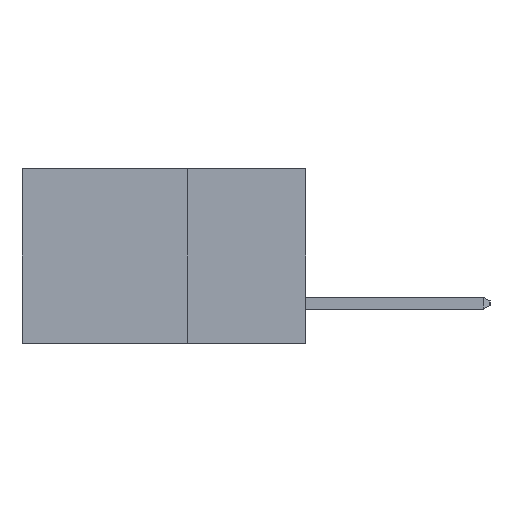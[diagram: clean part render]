
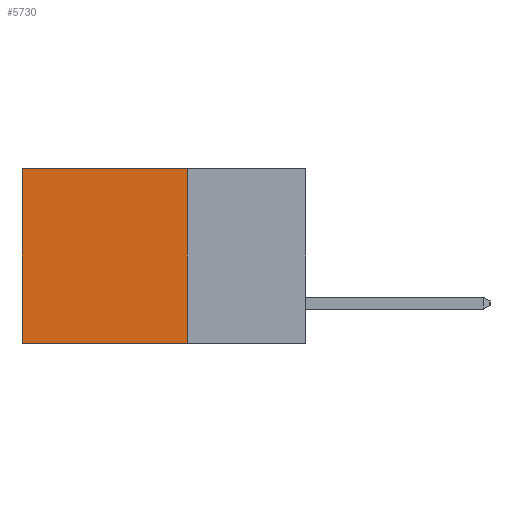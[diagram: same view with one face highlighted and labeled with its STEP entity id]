
A CAD part, left-side view. The second image highlights one B-rep face of the part: STEP entity #5730.
In plain terms, the highlighted planar face has unit normal (-1, 0, 0).
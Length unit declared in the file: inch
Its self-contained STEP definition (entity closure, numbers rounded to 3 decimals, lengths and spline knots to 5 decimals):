
#432 = ORIENTED_EDGE ( 'NONE', *, *, #12054, .F. ) ;
#1038 = EDGE_LOOP ( 'NONE', ( #14572, #3369, #432, #4384 ) ) ;
#1232 = CARTESIAN_POINT ( 'NONE',  ( 0.298, 0.25, 0. ) ) ;
#1444 = VECTOR ( 'NONE', #12503, 39.37008 ) ;
#2097 = CARTESIAN_POINT ( 'NONE',  ( 0.298, 0.6, -0.37 ) ) ;
#2151 = VERTEX_POINT ( 'NONE', #5497 ) ;
#2325 = LINE ( 'NONE', #1232, #12451 ) ;
#2976 = DIRECTION ( 'NONE',  ( 0., 0., -1. ) ) ;
#3150 = EDGE_CURVE ( 'NONE', #10001, #14254, #14470, .T. ) ;
#3329 = CARTESIAN_POINT ( 'NONE',  ( 0.298, 0.25, -0.37 ) ) ;
#3369 = ORIENTED_EDGE ( 'NONE', *, *, #3150, .F. ) ;
#4040 = CARTESIAN_POINT ( 'NONE',  ( 0.298, 0.25, 0. ) ) ;
#4271 = CARTESIAN_POINT ( 'NONE',  ( 0.298, 0.6, 0. ) ) ;
#4372 = DIRECTION ( 'NONE',  ( 1., 0., 0. ) ) ;
#4384 = ORIENTED_EDGE ( 'NONE', *, *, #6119, .T. ) ;
#5010 = LINE ( 'NONE', #4040, #14795 ) ;
#5497 = CARTESIAN_POINT ( 'NONE',  ( 0.298, 0.6, 0. ) ) ;
#5730 = ADVANCED_FACE ( 'NONE', ( #5785 ), #10461, .F. ) ;
#5785 = FACE_OUTER_BOUND ( 'NONE', #1038, .T. ) ;
#6119 = EDGE_CURVE ( 'NONE', #14207, #2151, #2325, .T. ) ;
#7699 = DIRECTION ( 'NONE',  ( 0., 0., -1. ) ) ;
#10001 = VERTEX_POINT ( 'NONE', #13879 ) ;
#10031 = DIRECTION ( 'NONE',  ( 0., 1., 0. ) ) ;
#10441 = CARTESIAN_POINT ( 'NONE',  ( 0.298, 0.25, 0. ) ) ;
#10461 = PLANE ( 'NONE',  #11547 ) ;
#11547 = AXIS2_PLACEMENT_3D ( 'NONE', #10441, #4372, #7699 ) ;
#12054 = EDGE_CURVE ( 'NONE', #14207, #10001, #5010, .T. ) ;
#12451 = VECTOR ( 'NONE', #10031, 39.37008 ) ;
#12478 = DIRECTION ( 'NONE',  ( 0., 0., -1. ) ) ;
#12503 = DIRECTION ( 'NONE',  ( 0., 1., 0. ) ) ;
#12982 = CARTESIAN_POINT ( 'NONE',  ( 0.298, 0.25, 0. ) ) ;
#13879 = CARTESIAN_POINT ( 'NONE',  ( 0.298, 0.25, -0.37 ) ) ;
#14207 = VERTEX_POINT ( 'NONE', #12982 ) ;
#14254 = VERTEX_POINT ( 'NONE', #2097 ) ;
#14470 = LINE ( 'NONE', #3329, #1444 ) ;
#14572 = ORIENTED_EDGE ( 'NONE', *, *, #14835, .T. ) ;
#14795 = VECTOR ( 'NONE', #12478, 39.37008 ) ;
#14835 = EDGE_CURVE ( 'NONE', #2151, #14254, #14887, .T. ) ;
#14887 = LINE ( 'NONE', #4271, #15267 ) ;
#15267 = VECTOR ( 'NONE', #2976, 39.37008 ) ;
